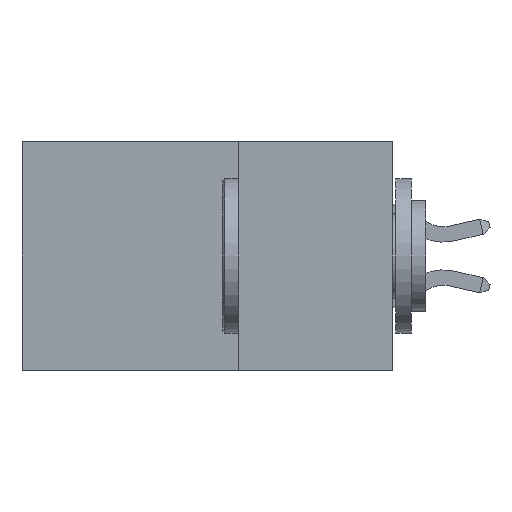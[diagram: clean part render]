
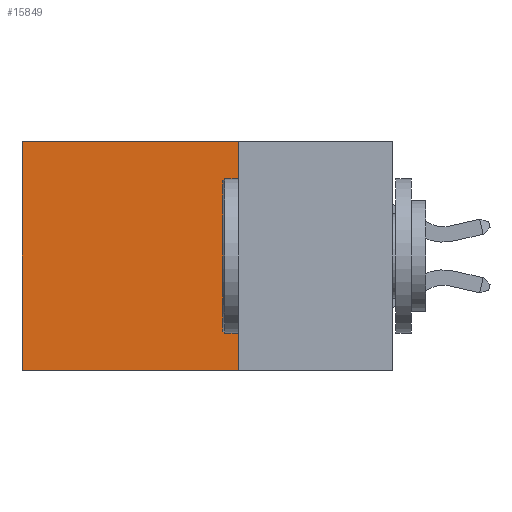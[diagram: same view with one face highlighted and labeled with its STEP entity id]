
A CAD part, left-side view. The second image highlights one B-rep face of the part: STEP entity #15849.
In plain terms, the highlighted planar face has unit normal (-1, 0, 0).
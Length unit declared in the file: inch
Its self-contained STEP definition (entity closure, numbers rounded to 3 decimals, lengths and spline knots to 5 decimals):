
#62 = EDGE_CURVE ( 'NONE', #17823, #13030, #11797, .T. ) ;
#108 = ORIENTED_EDGE ( 'NONE', *, *, #15021, .T. ) ;
#680 = CARTESIAN_POINT ( 'NONE',  ( 0.2875, 0.6, 0. ) ) ;
#926 = VECTOR ( 'NONE', #14162, 39.37008 ) ;
#1786 = DIRECTION ( 'NONE',  ( 0., 0., -1. ) ) ;
#1834 = ORIENTED_EDGE ( 'NONE', *, *, #62, .F. ) ;
#2002 = CARTESIAN_POINT ( 'NONE',  ( 0.2875, 0.25, 0. ) ) ;
#3051 = LINE ( 'NONE', #4998, #17515 ) ;
#3852 = CARTESIAN_POINT ( 'NONE',  ( 0.2875, 0.25, -0.37 ) ) ;
#4904 = EDGE_LOOP ( 'NONE', ( #10626, #1834, #6750, #108 ) ) ;
#4998 = CARTESIAN_POINT ( 'NONE',  ( 0.2875, 0.25, 0. ) ) ;
#5385 = EDGE_CURVE ( 'NONE', #13356, #17823, #3051, .T. ) ;
#5674 = CARTESIAN_POINT ( 'NONE',  ( 0.2875, 0.25, 0. ) ) ;
#5713 = CARTESIAN_POINT ( 'NONE',  ( 0.2875, 0.6, 0. ) ) ;
#6342 = CARTESIAN_POINT ( 'NONE',  ( 0.2875, 0.6, -0.37 ) ) ;
#6750 = ORIENTED_EDGE ( 'NONE', *, *, #5385, .F. ) ;
#7417 = VECTOR ( 'NONE', #17700, 39.37008 ) ;
#7467 = PLANE ( 'NONE',  #15722 ) ;
#7550 = CARTESIAN_POINT ( 'NONE',  ( 0.2875, 0.25, -0.37 ) ) ;
#8248 = LINE ( 'NONE', #5713, #926 ) ;
#9856 = EDGE_CURVE ( 'NONE', #13053, #13030, #8248, .T. ) ;
#10513 = LINE ( 'NONE', #2002, #17300 ) ;
#10626 = ORIENTED_EDGE ( 'NONE', *, *, #9856, .T. ) ;
#11736 = DIRECTION ( 'NONE',  ( 1., 0., 0. ) ) ;
#11797 = LINE ( 'NONE', #3852, #7417 ) ;
#11965 = DIRECTION ( 'NONE',  ( 0., 0., -1. ) ) ;
#13030 = VERTEX_POINT ( 'NONE', #6342 ) ;
#13053 = VERTEX_POINT ( 'NONE', #680 ) ;
#13181 = DIRECTION ( 'NONE',  ( 0., 1., 0. ) ) ;
#13356 = VERTEX_POINT ( 'NONE', #5674 ) ;
#14162 = DIRECTION ( 'NONE',  ( 0., 0., -1. ) ) ;
#14519 = CARTESIAN_POINT ( 'NONE',  ( 0.2875, 0.25, 0. ) ) ;
#15021 = EDGE_CURVE ( 'NONE', #13356, #13053, #10513, .T. ) ;
#15292 = FACE_OUTER_BOUND ( 'NONE', #4904, .T. ) ;
#15722 = AXIS2_PLACEMENT_3D ( 'NONE', #14519, #11736, #1786 ) ;
#15849 = ADVANCED_FACE ( 'NONE', ( #15292 ), #7467, .F. ) ;
#17300 = VECTOR ( 'NONE', #13181, 39.37008 ) ;
#17515 = VECTOR ( 'NONE', #11965, 39.37008 ) ;
#17700 = DIRECTION ( 'NONE',  ( 0., 1., 0. ) ) ;
#17823 = VERTEX_POINT ( 'NONE', #7550 ) ;
